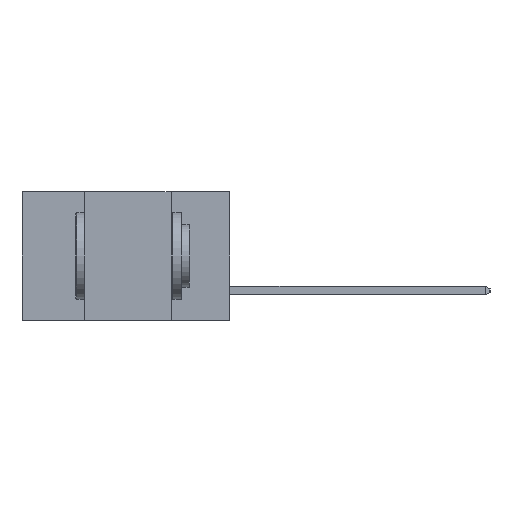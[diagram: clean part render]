
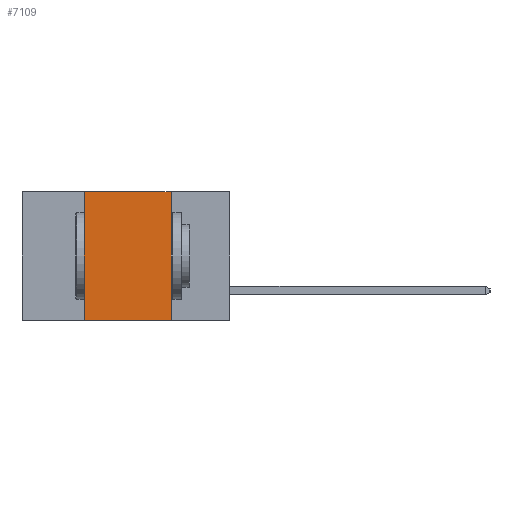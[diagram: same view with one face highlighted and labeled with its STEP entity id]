
A CAD part, left-side view. The second image highlights one B-rep face of the part: STEP entity #7109.
In plain terms, the highlighted planar face has unit normal (-1, 0, 0).
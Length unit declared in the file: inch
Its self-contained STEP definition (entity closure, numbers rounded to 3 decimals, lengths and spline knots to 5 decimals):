
#1361 = VECTOR ( 'NONE', #2292, 39.37008 ) ;
#2194 = LINE ( 'NONE', #8079, #14187 ) ;
#2292 = DIRECTION ( 'NONE',  ( 0., 0., -1. ) ) ;
#2626 = CARTESIAN_POINT ( 'NONE',  ( 0., 0.17, 0. ) ) ;
#2982 = EDGE_CURVE ( 'NONE', #20030, #12117, #11848, .T. ) ;
#5380 = EDGE_CURVE ( 'NONE', #12785, #21878, #18605, .T. ) ;
#7055 = CARTESIAN_POINT ( 'NONE',  ( 0., 0.42, -0.37 ) ) ;
#7109 = ADVANCED_FACE ( 'NONE', ( #15816 ), #22072, .F. ) ;
#7576 = CARTESIAN_POINT ( 'NONE',  ( 0., 0.42, 0. ) ) ;
#8079 = CARTESIAN_POINT ( 'NONE',  ( 0., 0.6, -0.37 ) ) ;
#11118 = DIRECTION ( 'NONE',  ( 1., 0., 0. ) ) ;
#11188 = EDGE_CURVE ( 'NONE', #12117, #12785, #28476, .T. ) ;
#11525 = EDGE_CURVE ( 'NONE', #20030, #21878, #2194, .T. ) ;
#11848 = LINE ( 'NONE', #7576, #17026 ) ;
#12117 = VERTEX_POINT ( 'NONE', #19001 ) ;
#12785 = VERTEX_POINT ( 'NONE', #25536 ) ;
#12793 = ORIENTED_EDGE ( 'NONE', *, *, #2982, .F. ) ;
#14187 = VECTOR ( 'NONE', #23477, 39.37008 ) ;
#15816 = FACE_OUTER_BOUND ( 'NONE', #26550, .T. ) ;
#16105 = AXIS2_PLACEMENT_3D ( 'NONE', #24284, #11118, #26435 ) ;
#16582 = ORIENTED_EDGE ( 'NONE', *, *, #5380, .F. ) ;
#17026 = VECTOR ( 'NONE', #20426, 39.37008 ) ;
#18605 = LINE ( 'NONE', #2626, #1361 ) ;
#19001 = CARTESIAN_POINT ( 'NONE',  ( 0., 0.42, 0. ) ) ;
#20030 = VERTEX_POINT ( 'NONE', #7055 ) ;
#20426 = DIRECTION ( 'NONE',  ( 0., 0., 1. ) ) ;
#21878 = VERTEX_POINT ( 'NONE', #22661 ) ;
#22072 = PLANE ( 'NONE',  #16105 ) ;
#22247 = CARTESIAN_POINT ( 'NONE',  ( 0., 0.6, 0. ) ) ;
#22661 = CARTESIAN_POINT ( 'NONE',  ( 0., 0.17, -0.37 ) ) ;
#23477 = DIRECTION ( 'NONE',  ( 0., -1., 0. ) ) ;
#24284 = CARTESIAN_POINT ( 'NONE',  ( 0., 0.6, 0. ) ) ;
#24460 = DIRECTION ( 'NONE',  ( 0., -1., 0. ) ) ;
#25536 = CARTESIAN_POINT ( 'NONE',  ( 0., 0.17, 0. ) ) ;
#25830 = ORIENTED_EDGE ( 'NONE', *, *, #11525, .T. ) ;
#26435 = DIRECTION ( 'NONE',  ( 0., 0., -1. ) ) ;
#26550 = EDGE_LOOP ( 'NONE', ( #16582, #28103, #12793, #25830 ) ) ;
#27839 = VECTOR ( 'NONE', #24460, 39.37008 ) ;
#28103 = ORIENTED_EDGE ( 'NONE', *, *, #11188, .F. ) ;
#28476 = LINE ( 'NONE', #22247, #27839 ) ;
